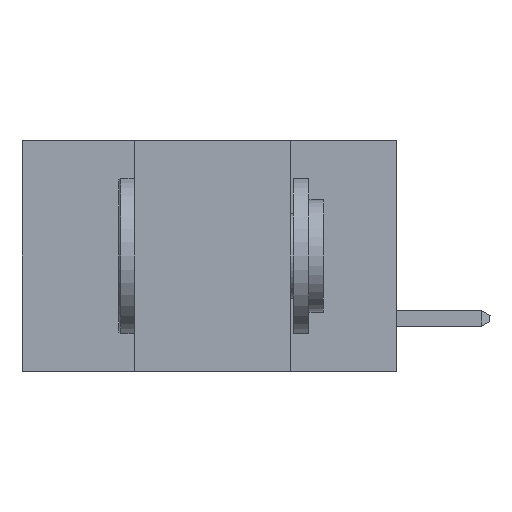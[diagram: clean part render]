
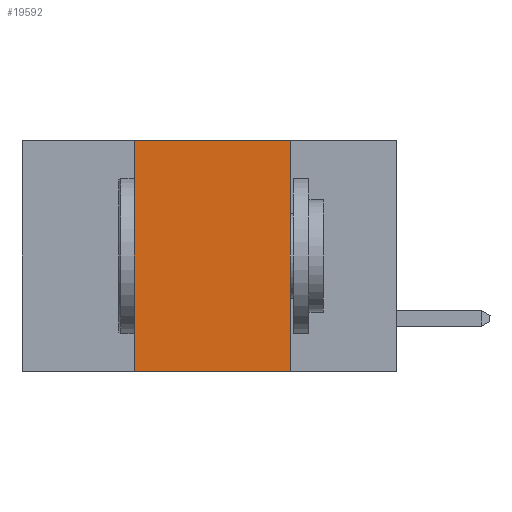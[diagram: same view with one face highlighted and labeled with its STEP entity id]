
A CAD part, left-side view. The second image highlights one B-rep face of the part: STEP entity #19592.
In plain terms, the highlighted planar face has unit normal (-1, 0, 0).
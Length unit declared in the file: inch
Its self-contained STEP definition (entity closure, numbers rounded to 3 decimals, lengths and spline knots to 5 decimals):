
#230 = VERTEX_POINT ( 'NONE', #13703 ) ;
#529 = LINE ( 'NONE', #20543, #26165 ) ;
#919 = VERTEX_POINT ( 'NONE', #25221 ) ;
#2594 = DIRECTION ( 'NONE',  ( 0., 0., -1. ) ) ;
#3466 = VECTOR ( 'NONE', #2594, 39.37008 ) ;
#3476 = DIRECTION ( 'NONE',  ( 1., 0., 0. ) ) ;
#3841 = PLANE ( 'NONE',  #10710 ) ;
#5464 = ORIENTED_EDGE ( 'NONE', *, *, #7061, .T. ) ;
#5484 = CARTESIAN_POINT ( 'NONE',  ( 0., 0.6, -0.37 ) ) ;
#6110 = LINE ( 'NONE', #13037, #9987 ) ;
#6492 = EDGE_CURVE ( 'NONE', #230, #9549, #529, .T. ) ;
#7061 = EDGE_CURVE ( 'NONE', #230, #919, #17798, .T. ) ;
#7254 = DIRECTION ( 'NONE',  ( 0., -1., 0. ) ) ;
#9549 = VERTEX_POINT ( 'NONE', #22717 ) ;
#9987 = VECTOR ( 'NONE', #12941, 39.37008 ) ;
#10060 = FACE_OUTER_BOUND ( 'NONE', #22825, .T. ) ;
#10710 = AXIS2_PLACEMENT_3D ( 'NONE', #15726, #3476, #24404 ) ;
#12301 = ORIENTED_EDGE ( 'NONE', *, *, #6492, .F. ) ;
#12310 = EDGE_CURVE ( 'NONE', #20793, #919, #16278, .T. ) ;
#12941 = DIRECTION ( 'NONE',  ( 0., -1., 0. ) ) ;
#13037 = CARTESIAN_POINT ( 'NONE',  ( 0., 0.6, 0. ) ) ;
#13391 = CARTESIAN_POINT ( 'NONE',  ( 0., 0.17, 0. ) ) ;
#13703 = CARTESIAN_POINT ( 'NONE',  ( 0., 0.42, -0.37 ) ) ;
#14218 = DIRECTION ( 'NONE',  ( 0., 0., 1. ) ) ;
#15726 = CARTESIAN_POINT ( 'NONE',  ( 0., 0.6, 0. ) ) ;
#16278 = LINE ( 'NONE', #24976, #3466 ) ;
#16495 = VECTOR ( 'NONE', #7254, 39.37008 ) ;
#17798 = LINE ( 'NONE', #5484, #16495 ) ;
#19592 = ADVANCED_FACE ( 'NONE', ( #10060 ), #3841, .F. ) ;
#20543 = CARTESIAN_POINT ( 'NONE',  ( 0., 0.42, 0. ) ) ;
#20647 = EDGE_CURVE ( 'NONE', #9549, #20793, #6110, .T. ) ;
#20793 = VERTEX_POINT ( 'NONE', #13391 ) ;
#22110 = ORIENTED_EDGE ( 'NONE', *, *, #20647, .F. ) ;
#22717 = CARTESIAN_POINT ( 'NONE',  ( 0., 0.42, 0. ) ) ;
#22825 = EDGE_LOOP ( 'NONE', ( #25740, #22110, #12301, #5464 ) ) ;
#24404 = DIRECTION ( 'NONE',  ( 0., 0., -1. ) ) ;
#24976 = CARTESIAN_POINT ( 'NONE',  ( 0., 0.17, 0. ) ) ;
#25221 = CARTESIAN_POINT ( 'NONE',  ( 0., 0.17, -0.37 ) ) ;
#25740 = ORIENTED_EDGE ( 'NONE', *, *, #12310, .F. ) ;
#26165 = VECTOR ( 'NONE', #14218, 39.37008 ) ;
